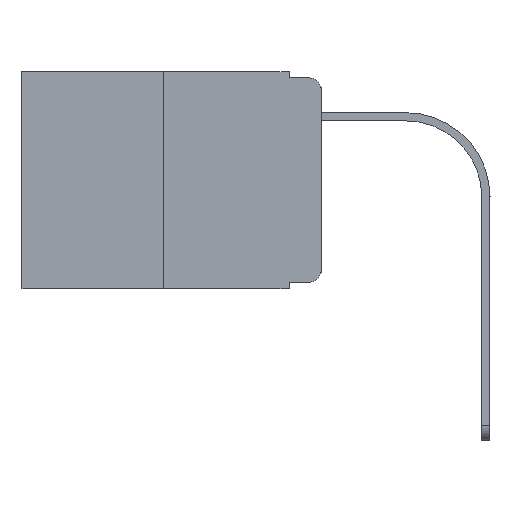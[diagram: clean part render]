
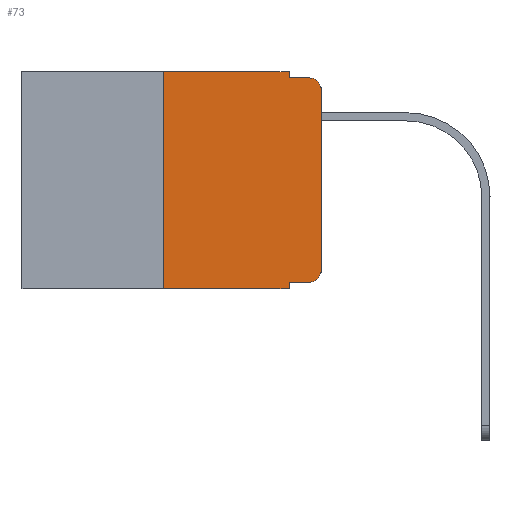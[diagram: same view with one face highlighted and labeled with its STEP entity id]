
A CAD part, left-side view. The second image highlights one B-rep face of the part: STEP entity #73.
In plain terms, the highlighted planar face has unit normal (-1, 0, 0).
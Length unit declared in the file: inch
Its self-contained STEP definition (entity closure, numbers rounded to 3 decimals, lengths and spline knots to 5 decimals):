
#22 = VERTEX_POINT ( 'NONE', #2807 ) ;
#73 = ADVANCED_FACE ( 'NONE', ( #3917 ), #637, .F. ) ;
#219 = CARTESIAN_POINT ( 'NONE',  ( 0., 0.051, -0.343 ) ) ;
#432 = LINE ( 'NONE', #6392, #11711 ) ;
#552 = CARTESIAN_POINT ( 'NONE',  ( 0., 0.051, -0.01 ) ) ;
#637 = PLANE ( 'NONE',  #4858 ) ;
#657 = CARTESIAN_POINT ( 'NONE',  ( 0., 0., -0.313 ) ) ;
#762 = DIRECTION ( 'NONE',  ( 0., 0., 1. ) ) ;
#771 = CARTESIAN_POINT ( 'NONE',  ( 0., 0.02, -0.333 ) ) ;
#890 = VECTOR ( 'NONE', #762, 39.37008 ) ;
#896 = VERTEX_POINT ( 'NONE', #13524 ) ;
#916 = CARTESIAN_POINT ( 'NONE',  ( 0., 0.25, 0. ) ) ;
#996 = LINE ( 'NONE', #916, #12819 ) ;
#1066 = ORIENTED_EDGE ( 'NONE', *, *, #6414, .F. ) ;
#1177 = DIRECTION ( 'NONE',  ( -1., 0., 0. ) ) ;
#1179 = EDGE_CURVE ( 'NONE', #7307, #896, #8211, .T. ) ;
#1427 = EDGE_CURVE ( 'NONE', #9274, #7307, #2955, .T. ) ;
#1449 = CARTESIAN_POINT ( 'NONE',  ( 0., 0.02, -0.03 ) ) ;
#1790 = EDGE_CURVE ( 'NONE', #2555, #9274, #2776, .T. ) ;
#2555 = VERTEX_POINT ( 'NONE', #5082 ) ;
#2718 = EDGE_CURVE ( 'NONE', #2555, #7476, #13535, .T. ) ;
#2751 = CARTESIAN_POINT ( 'NONE',  ( 0., 0.051, -0.01 ) ) ;
#2776 = LINE ( 'NONE', #3674, #4701 ) ;
#2786 = ORIENTED_EDGE ( 'NONE', *, *, #13167, .T. ) ;
#2807 = CARTESIAN_POINT ( 'NONE',  ( 0., 0.051, 0. ) ) ;
#2955 = CIRCLE ( 'NONE', #10760, 0.02 ) ;
#2960 = ORIENTED_EDGE ( 'NONE', *, *, #1790, .T. ) ;
#3480 = CARTESIAN_POINT ( 'NONE',  ( 0., 0.25, -0.343 ) ) ;
#3674 = CARTESIAN_POINT ( 'NONE',  ( 0., 0.051, -0.333 ) ) ;
#3734 = EDGE_CURVE ( 'NONE', #4832, #10388, #996, .T. ) ;
#3767 = CIRCLE ( 'NONE', #8445, 0.02 ) ;
#3917 = FACE_OUTER_BOUND ( 'NONE', #13228, .T. ) ;
#4028 = DIRECTION ( 'NONE',  ( 0., 0., -1. ) ) ;
#4057 = CARTESIAN_POINT ( 'NONE',  ( 0., 0.02, -0.01 ) ) ;
#4557 = EDGE_CURVE ( 'NONE', #10388, #22, #432, .T. ) ;
#4701 = VECTOR ( 'NONE', #7022, 39.37008 ) ;
#4832 = VERTEX_POINT ( 'NONE', #3480 ) ;
#4858 = AXIS2_PLACEMENT_3D ( 'NONE', #4869, #9143, #13440 ) ;
#4869 = CARTESIAN_POINT ( 'NONE',  ( 0., 0.473, 0. ) ) ;
#4882 = ORIENTED_EDGE ( 'NONE', *, *, #2718, .F. ) ;
#5082 = CARTESIAN_POINT ( 'NONE',  ( 0., 0.051, -0.333 ) ) ;
#5404 = DIRECTION ( 'NONE',  ( 0., 0., -1. ) ) ;
#5755 = ORIENTED_EDGE ( 'NONE', *, *, #9215, .T. ) ;
#6392 = CARTESIAN_POINT ( 'NONE',  ( 0., 0.473, 0. ) ) ;
#6414 = EDGE_CURVE ( 'NONE', #22, #13597, #9273, .T. ) ;
#6465 = VECTOR ( 'NONE', #7946, 39.37008 ) ;
#6493 = ORIENTED_EDGE ( 'NONE', *, *, #7305, .F. ) ;
#6998 = DIRECTION ( 'NONE',  ( 0., -1., 0. ) ) ;
#7002 = VECTOR ( 'NONE', #4028, 39.37008 ) ;
#7022 = DIRECTION ( 'NONE',  ( 0., -1., 0. ) ) ;
#7305 = EDGE_CURVE ( 'NONE', #13597, #8840, #12332, .T. ) ;
#7307 = VERTEX_POINT ( 'NONE', #657 ) ;
#7387 = DIRECTION ( 'NONE',  ( 0., 0., 1. ) ) ;
#7476 = VERTEX_POINT ( 'NONE', #219 ) ;
#7867 = ORIENTED_EDGE ( 'NONE', *, *, #1427, .T. ) ;
#7946 = DIRECTION ( 'NONE',  ( 0., -1., 0. ) ) ;
#8211 = LINE ( 'NONE', #9271, #890 ) ;
#8336 = ORIENTED_EDGE ( 'NONE', *, *, #3734, .F. ) ;
#8445 = AXIS2_PLACEMENT_3D ( 'NONE', #1449, #9954, #13193 ) ;
#8623 = CARTESIAN_POINT ( 'NONE',  ( 0., 0.02, -0.313 ) ) ;
#8840 = VERTEX_POINT ( 'NONE', #4057 ) ;
#9143 = DIRECTION ( 'NONE',  ( 1., 0., 0. ) ) ;
#9215 = EDGE_CURVE ( 'NONE', #4832, #7476, #13297, .T. ) ;
#9271 = CARTESIAN_POINT ( 'NONE',  ( 0., 0., 0. ) ) ;
#9273 = LINE ( 'NONE', #10454, #7002 ) ;
#9274 = VERTEX_POINT ( 'NONE', #771 ) ;
#9387 = DIRECTION ( 'NONE',  ( 0., 0., -1. ) ) ;
#9486 = DIRECTION ( 'NONE',  ( 0., -1., 0. ) ) ;
#9764 = ORIENTED_EDGE ( 'NONE', *, *, #1179, .T. ) ;
#9866 = VECTOR ( 'NONE', #9387, 39.37008 ) ;
#9954 = DIRECTION ( 'NONE',  ( -1., 0., 0. ) ) ;
#10388 = VERTEX_POINT ( 'NONE', #12610 ) ;
#10454 = CARTESIAN_POINT ( 'NONE',  ( 0., 0.051, 0. ) ) ;
#10760 = AXIS2_PLACEMENT_3D ( 'NONE', #8623, #1177, #5404 ) ;
#11711 = VECTOR ( 'NONE', #9486, 39.37008 ) ;
#12302 = ORIENTED_EDGE ( 'NONE', *, *, #4557, .F. ) ;
#12332 = LINE ( 'NONE', #2751, #12994 ) ;
#12610 = CARTESIAN_POINT ( 'NONE',  ( 0., 0.25, 0. ) ) ;
#12819 = VECTOR ( 'NONE', #7387, 39.37008 ) ;
#12994 = VECTOR ( 'NONE', #6998, 39.37008 ) ;
#13018 = CARTESIAN_POINT ( 'NONE',  ( 0., 0.473, -0.343 ) ) ;
#13167 = EDGE_CURVE ( 'NONE', #896, #8840, #3767, .T. ) ;
#13193 = DIRECTION ( 'NONE',  ( 0., 0., -1. ) ) ;
#13228 = EDGE_LOOP ( 'NONE', ( #9764, #2786, #6493, #1066, #12302, #8336, #5755, #4882, #2960, #7867 ) ) ;
#13297 = LINE ( 'NONE', #13018, #6465 ) ;
#13440 = DIRECTION ( 'NONE',  ( 0., 0., -1. ) ) ;
#13524 = CARTESIAN_POINT ( 'NONE',  ( 0., 0., -0.03 ) ) ;
#13535 = LINE ( 'NONE', #13737, #9866 ) ;
#13597 = VERTEX_POINT ( 'NONE', #552 ) ;
#13737 = CARTESIAN_POINT ( 'NONE',  ( 0., 0.051, 0. ) ) ;
